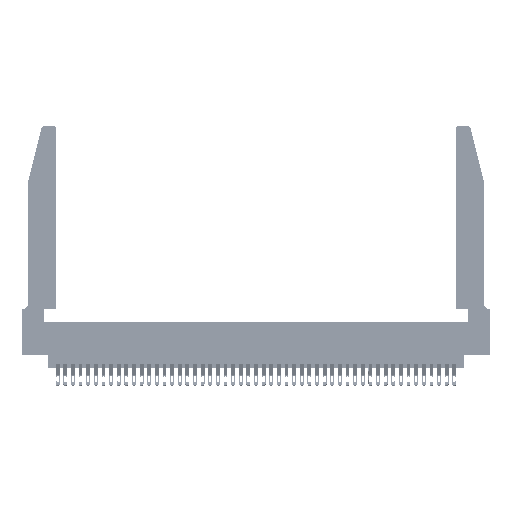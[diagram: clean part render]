
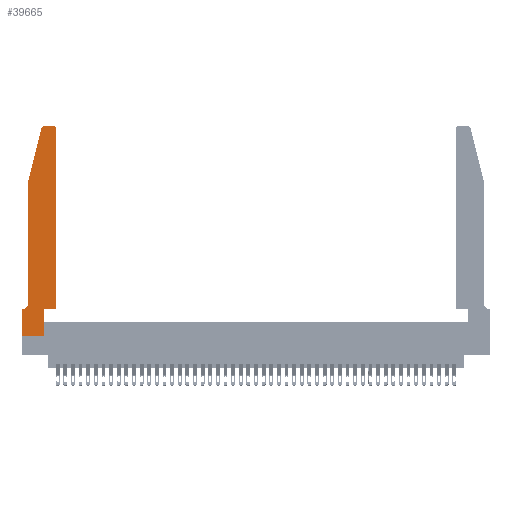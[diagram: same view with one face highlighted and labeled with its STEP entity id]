
A CAD part, top view. The second image highlights one B-rep face of the part: STEP entity #39665.
In plain terms, the highlighted planar face has unit normal (0, 0, 1).
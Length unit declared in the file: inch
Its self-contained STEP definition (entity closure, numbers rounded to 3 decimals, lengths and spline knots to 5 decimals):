
#151 = VECTOR ( 'NONE', #31217, 39.37008 ) ;
#605 = PLANE ( 'NONE',  #14400 ) ;
#757 = VECTOR ( 'NONE', #12105, 39.37008 ) ;
#1443 = LINE ( 'NONE', #31695, #10233 ) ;
#2122 = CARTESIAN_POINT ( 'NONE',  ( 0.0755, 0.35, 0.37 ) ) ;
#2634 = EDGE_CURVE ( 'NONE', #33338, #42551, #41855, .T. ) ;
#3232 = AXIS2_PLACEMENT_3D ( 'NONE', #6215, #10350, #41733 ) ;
#4758 = CARTESIAN_POINT ( 'NONE',  ( 0., 0., 0.37 ) ) ;
#5529 = CARTESIAN_POINT ( 'NONE',  ( 0.0055, 0.35, 0.37 ) ) ;
#5787 = LINE ( 'NONE', #29528, #757 ) ;
#6103 = EDGE_CURVE ( 'NONE', #29384, #25986, #16712, .T. ) ;
#6215 = CARTESIAN_POINT ( 'NONE',  ( 0.4205, 2.72, 0.37 ) ) ;
#7279 = VERTEX_POINT ( 'NONE', #5529 ) ;
#7709 = DIRECTION ( 'NONE',  ( 0., 0., 1. ) ) ;
#8268 = CARTESIAN_POINT ( 'NONE',  ( 0., 0., 0.37 ) ) ;
#8403 = CARTESIAN_POINT ( 'NONE',  ( 0.4205, 2.75, 0.37 ) ) ;
#8422 = LINE ( 'NONE', #2122, #28636 ) ;
#9369 = VERTEX_POINT ( 'NONE', #8403 ) ;
#10233 = VECTOR ( 'NONE', #36129, 39.37008 ) ;
#10350 = DIRECTION ( 'NONE',  ( 0., 0., 1. ) ) ;
#10669 = EDGE_CURVE ( 'NONE', #42551, #39666, #1443, .T. ) ;
#11399 = CARTESIAN_POINT ( 'NONE',  ( 0., 0.35, 0.37 ) ) ;
#11473 = ORIENTED_EDGE ( 'NONE', *, *, #6103, .T. ) ;
#11617 = ORIENTED_EDGE ( 'NONE', *, *, #18417, .T. ) ;
#11944 = DIRECTION ( 'NONE',  ( 0., -1., 0. ) ) ;
#12105 = DIRECTION ( 'NONE',  ( 0., 1., 0. ) ) ;
#13053 = EDGE_CURVE ( 'NONE', #22373, #42423, #34141, .T. ) ;
#13316 = CARTESIAN_POINT ( 'NONE',  ( 0.284, 2.72, 0.37 ) ) ;
#13559 = DIRECTION ( 'NONE',  ( 0., 0., -1. ) ) ;
#13838 = CIRCLE ( 'NONE', #23703, 0.07 ) ;
#14400 = AXIS2_PLACEMENT_3D ( 'NONE', #42463, #7709, #28392 ) ;
#14733 = ORIENTED_EDGE ( 'NONE', *, *, #13053, .T. ) ;
#14870 = ORIENTED_EDGE ( 'NONE', *, *, #16868, .T. ) ;
#16386 = ORIENTED_EDGE ( 'NONE', *, *, #19647, .T. ) ;
#16712 = LINE ( 'NONE', #8268, #36885 ) ;
#16868 = EDGE_CURVE ( 'NONE', #42423, #9369, #31551, .T. ) ;
#17053 = ORIENTED_EDGE ( 'NONE', *, *, #38838, .T. ) ;
#17210 = CARTESIAN_POINT ( 'NONE',  ( 0.0755, 2., 0.37 ) ) ;
#17676 = ORIENTED_EDGE ( 'NONE', *, *, #2634, .T. ) ;
#17801 = VECTOR ( 'NONE', #35510, 39.37008 ) ;
#18417 = EDGE_CURVE ( 'NONE', #23529, #31681, #5787, .T. ) ;
#18695 = EDGE_CURVE ( 'NONE', #9369, #38546, #44130, .T. ) ;
#18967 = CARTESIAN_POINT ( 'NONE',  ( 0.4505, 2.72, 0.37 ) ) ;
#19102 = EDGE_CURVE ( 'NONE', #31681, #22373, #34477, .T. ) ;
#19222 = CARTESIAN_POINT ( 'NONE',  ( 0.4505, 0.35, 0.37 ) ) ;
#19274 = CARTESIAN_POINT ( 'NONE',  ( 0.0755, 2., 0.37 ) ) ;
#19630 = CARTESIAN_POINT ( 'NONE',  ( 0.0055, 0.42, 0.37 ) ) ;
#19647 = EDGE_CURVE ( 'NONE', #25986, #23529, #38876, .T. ) ;
#19784 = VECTOR ( 'NONE', #39484, 39.37008 ) ;
#21464 = CARTESIAN_POINT ( 'NONE',  ( 0., 0., 0.37 ) ) ;
#21490 = EDGE_CURVE ( 'NONE', #38546, #33338, #31589, .T. ) ;
#21534 = VECTOR ( 'NONE', #42475, 39.37008 ) ;
#22373 = VERTEX_POINT ( 'NONE', #44361 ) ;
#23525 = DIRECTION ( 'NONE',  ( 1., 0., 0. ) ) ;
#23529 = VERTEX_POINT ( 'NONE', #24589 ) ;
#23703 = AXIS2_PLACEMENT_3D ( 'NONE', #19630, #13559, #41538 ) ;
#23811 = ORIENTED_EDGE ( 'NONE', *, *, #10669, .T. ) ;
#23987 = CARTESIAN_POINT ( 'NONE',  ( 0.4505, 0.35, 0.37 ) ) ;
#24545 = CARTESIAN_POINT ( 'NONE',  ( 0.0755, 0.42, 0.37 ) ) ;
#24569 = EDGE_CURVE ( 'NONE', #39666, #7279, #13838, .T. ) ;
#24589 = CARTESIAN_POINT ( 'NONE',  ( 0.2865, 0., 0.37 ) ) ;
#25986 = VERTEX_POINT ( 'NONE', #21464 ) ;
#28392 = DIRECTION ( 'NONE',  ( 1., 0., 0. ) ) ;
#28497 = VECTOR ( 'NONE', #43738, 39.37008 ) ;
#28636 = VECTOR ( 'NONE', #37185, 39.37008 ) ;
#29384 = VERTEX_POINT ( 'NONE', #11399 ) ;
#29528 = CARTESIAN_POINT ( 'NONE',  ( 0.2865, 0.35, 0.37 ) ) ;
#29651 = CARTESIAN_POINT ( 'NONE',  ( 0.25487, 2.72718, 0.37 ) ) ;
#31217 = DIRECTION ( 'NONE',  ( -0.239, -0.971, 0. ) ) ;
#31247 = EDGE_LOOP ( 'NONE', ( #42172, #43760, #17676, #23811, #32850, #17053, #11473, #16386, #11617, #31298, #14733, #14870 ) ) ;
#31298 = ORIENTED_EDGE ( 'NONE', *, *, #19102, .T. ) ;
#31551 = CIRCLE ( 'NONE', #3232, 0.03 ) ;
#31589 = CIRCLE ( 'NONE', #37980, 0.03 ) ;
#31681 = VERTEX_POINT ( 'NONE', #42422 ) ;
#31695 = CARTESIAN_POINT ( 'NONE',  ( 0.0755, 2., 0.37 ) ) ;
#32411 = CARTESIAN_POINT ( 'NONE',  ( 0.284, 2.75, 0.37 ) ) ;
#32850 = ORIENTED_EDGE ( 'NONE', *, *, #24569, .T. ) ;
#33338 = VERTEX_POINT ( 'NONE', #29651 ) ;
#34141 = LINE ( 'NONE', #23987, #21534 ) ;
#34477 = LINE ( 'NONE', #19222, #28497 ) ;
#35510 = DIRECTION ( 'NONE',  ( -1., 0., 0. ) ) ;
#36129 = DIRECTION ( 'NONE',  ( 0., -1., 0. ) ) ;
#36885 = VECTOR ( 'NONE', #11944, 39.37008 ) ;
#37185 = DIRECTION ( 'NONE',  ( -1., 0., 0. ) ) ;
#37606 = DIRECTION ( 'NONE',  ( 0., 0., 1. ) ) ;
#37980 = AXIS2_PLACEMENT_3D ( 'NONE', #13316, #37606, #23525 ) ;
#38546 = VERTEX_POINT ( 'NONE', #32411 ) ;
#38838 = EDGE_CURVE ( 'NONE', #7279, #29384, #8422, .T. ) ;
#38876 = LINE ( 'NONE', #4758, #19784 ) ;
#39484 = DIRECTION ( 'NONE',  ( 1., 0., 0. ) ) ;
#39665 = ADVANCED_FACE ( 'NONE', ( #43962 ), #605, .T. ) ;
#39666 = VERTEX_POINT ( 'NONE', #24545 ) ;
#41538 = DIRECTION ( 'NONE',  ( -1., 0., 0. ) ) ;
#41733 = DIRECTION ( 'NONE',  ( 1., 0., 0. ) ) ;
#41855 = LINE ( 'NONE', #17210, #151 ) ;
#41876 = CARTESIAN_POINT ( 'NONE',  ( 0.2605, 2.75, 0.37 ) ) ;
#42172 = ORIENTED_EDGE ( 'NONE', *, *, #18695, .T. ) ;
#42422 = CARTESIAN_POINT ( 'NONE',  ( 0.2865, 0.35, 0.37 ) ) ;
#42423 = VERTEX_POINT ( 'NONE', #18967 ) ;
#42463 = CARTESIAN_POINT ( 'NONE',  ( 0., 0.35, 0.37 ) ) ;
#42475 = DIRECTION ( 'NONE',  ( 0., 1., 0. ) ) ;
#42551 = VERTEX_POINT ( 'NONE', #19274 ) ;
#43738 = DIRECTION ( 'NONE',  ( 1., 0., 0. ) ) ;
#43760 = ORIENTED_EDGE ( 'NONE', *, *, #21490, .T. ) ;
#43962 = FACE_OUTER_BOUND ( 'NONE', #31247, .T. ) ;
#44130 = LINE ( 'NONE', #41876, #17801 ) ;
#44361 = CARTESIAN_POINT ( 'NONE',  ( 0.4505, 0.35, 0.37 ) ) ;
